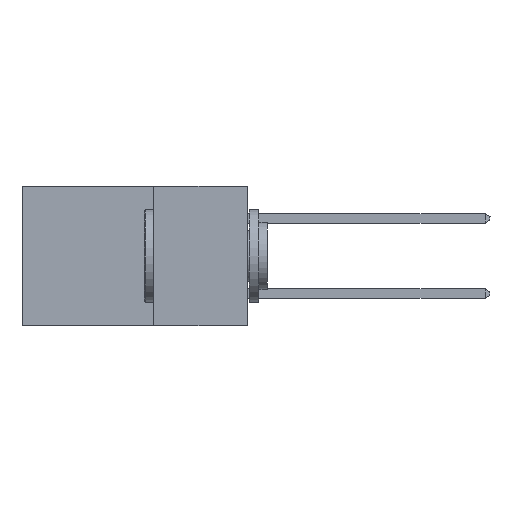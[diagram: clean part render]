
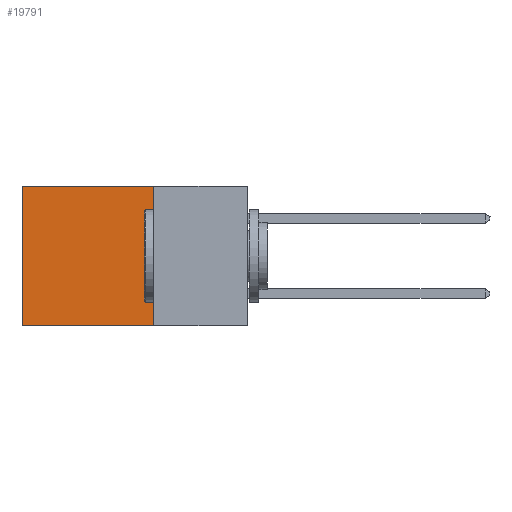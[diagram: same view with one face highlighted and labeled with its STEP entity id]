
A CAD part, left-side view. The second image highlights one B-rep face of the part: STEP entity #19791.
In plain terms, the highlighted planar face has unit normal (-1, 0, 0).
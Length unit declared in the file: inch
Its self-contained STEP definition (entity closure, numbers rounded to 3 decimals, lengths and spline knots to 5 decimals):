
#193 = DIRECTION ( 'NONE',  ( 0., 0., -1. ) ) ;
#534 = ORIENTED_EDGE ( 'NONE', *, *, #4798, .F. ) ;
#2014 = ORIENTED_EDGE ( 'NONE', *, *, #6021, .F. ) ;
#4017 = VERTEX_POINT ( 'NONE', #24725 ) ;
#4798 = EDGE_CURVE ( 'NONE', #4017, #22055, #21961, .T. ) ;
#6021 = EDGE_CURVE ( 'NONE', #22055, #7141, #21717, .T. ) ;
#7141 = VERTEX_POINT ( 'NONE', #20423 ) ;
#7527 = VERTEX_POINT ( 'NONE', #16425 ) ;
#7609 = VECTOR ( 'NONE', #22096, 39.37008 ) ;
#9146 = DIRECTION ( 'NONE',  ( 0., 1., 0. ) ) ;
#9660 = CARTESIAN_POINT ( 'NONE',  ( 0.2615, 0.25, -0.37 ) ) ;
#10396 = EDGE_CURVE ( 'NONE', #4017, #7527, #18731, .T. ) ;
#10561 = PLANE ( 'NONE',  #26420 ) ;
#11867 = ORIENTED_EDGE ( 'NONE', *, *, #14713, .T. ) ;
#12203 = CARTESIAN_POINT ( 'NONE',  ( 0.2615, 0.25, -0.37 ) ) ;
#12607 = DIRECTION ( 'NONE',  ( 1., 0., 0. ) ) ;
#14220 = FACE_OUTER_BOUND ( 'NONE', #17201, .T. ) ;
#14685 = CARTESIAN_POINT ( 'NONE',  ( 0.2615, 0.25, 0. ) ) ;
#14713 = EDGE_CURVE ( 'NONE', #7527, #7141, #22736, .T. ) ;
#15501 = CARTESIAN_POINT ( 'NONE',  ( 0.2615, 0.25, -0.37 ) ) ;
#15999 = VECTOR ( 'NONE', #9146, 39.37008 ) ;
#16381 = DIRECTION ( 'NONE',  ( 0., 0., -1. ) ) ;
#16425 = CARTESIAN_POINT ( 'NONE',  ( 0.2615, 0.6, 0. ) ) ;
#16510 = CARTESIAN_POINT ( 'NONE',  ( 0.2615, 0.6, -0.37 ) ) ;
#17201 = EDGE_LOOP ( 'NONE', ( #11867, #2014, #534, #20164 ) ) ;
#18343 = CARTESIAN_POINT ( 'NONE',  ( 0.2615, 0.25, -0.37 ) ) ;
#18731 = LINE ( 'NONE', #14685, #24910 ) ;
#19791 = ADVANCED_FACE ( 'NONE', ( #14220 ), #10561, .F. ) ;
#20164 = ORIENTED_EDGE ( 'NONE', *, *, #10396, .T. ) ;
#20423 = CARTESIAN_POINT ( 'NONE',  ( 0.2615, 0.6, -0.37 ) ) ;
#20913 = DIRECTION ( 'NONE',  ( 0., 1., 0. ) ) ;
#21552 = VECTOR ( 'NONE', #16381, 39.37008 ) ;
#21717 = LINE ( 'NONE', #15501, #15999 ) ;
#21961 = LINE ( 'NONE', #9660, #7609 ) ;
#22055 = VERTEX_POINT ( 'NONE', #18343 ) ;
#22096 = DIRECTION ( 'NONE',  ( 0., 0., -1. ) ) ;
#22736 = LINE ( 'NONE', #16510, #21552 ) ;
#24725 = CARTESIAN_POINT ( 'NONE',  ( 0.2615, 0.25, 0. ) ) ;
#24910 = VECTOR ( 'NONE', #20913, 39.37008 ) ;
#26420 = AXIS2_PLACEMENT_3D ( 'NONE', #12203, #12607, #193 ) ;
